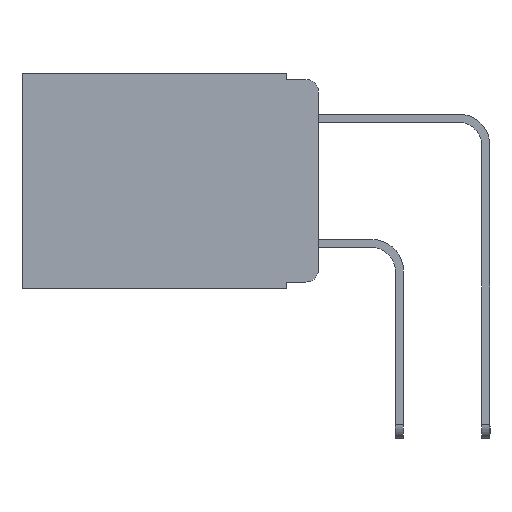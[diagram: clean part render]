
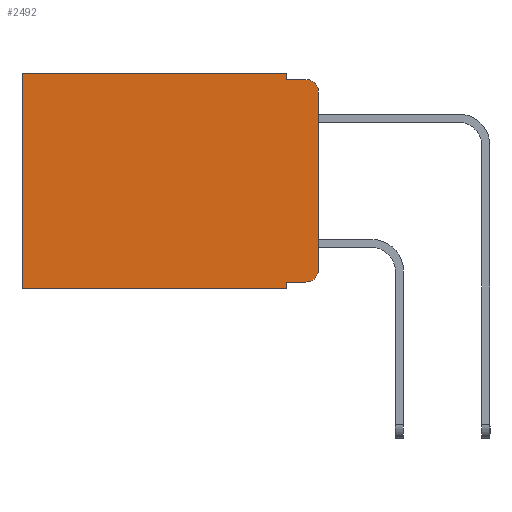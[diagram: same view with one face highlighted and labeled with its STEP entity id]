
A CAD part, left-side view. The second image highlights one B-rep face of the part: STEP entity #2492.
In plain terms, the highlighted planar face has unit normal (-1, 0, 0).
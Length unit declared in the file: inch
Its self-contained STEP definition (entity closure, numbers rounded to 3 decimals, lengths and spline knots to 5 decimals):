
#73 = ORIENTED_EDGE ( 'NONE', *, *, #131, .T. ) ;
#131 = EDGE_CURVE ( 'NONE', #2757, #17905, #5241, .T. ) ;
#643 = ORIENTED_EDGE ( 'NONE', *, *, #13208, .F. ) ;
#652 = CIRCLE ( 'NONE', #2332, 0.02 ) ;
#674 = VECTOR ( 'NONE', #5811, 39.37008 ) ;
#1659 = DIRECTION ( 'NONE',  ( 0., 0., -1. ) ) ;
#1940 = CARTESIAN_POINT ( 'NONE',  ( 0.298, 0.473, -0.343 ) ) ;
#2267 = ORIENTED_EDGE ( 'NONE', *, *, #25690, .F. ) ;
#2271 = ORIENTED_EDGE ( 'NONE', *, *, #12201, .T. ) ;
#2332 = AXIS2_PLACEMENT_3D ( 'NONE', #17751, #13495, #1659 ) ;
#2370 = ORIENTED_EDGE ( 'NONE', *, *, #26074, .T. ) ;
#2492 = ADVANCED_FACE ( 'NONE', ( #12790 ), #24912, .F. ) ;
#2679 = VERTEX_POINT ( 'NONE', #11055 ) ;
#2757 = VERTEX_POINT ( 'NONE', #25828 ) ;
#3081 = LINE ( 'NONE', #25718, #4951 ) ;
#3524 = VERTEX_POINT ( 'NONE', #13627 ) ;
#3707 = LINE ( 'NONE', #10097, #674 ) ;
#3813 = VECTOR ( 'NONE', #19562, 39.37008 ) ;
#3840 = CARTESIAN_POINT ( 'NONE',  ( 0.298, 0.051, -0.333 ) ) ;
#4006 = VECTOR ( 'NONE', #13855, 39.37008 ) ;
#4181 = CARTESIAN_POINT ( 'NONE',  ( 0.298, 0.051, -0.01 ) ) ;
#4200 = DIRECTION ( 'NONE',  ( 0., 0., -1. ) ) ;
#4491 = CARTESIAN_POINT ( 'NONE',  ( 0.298, 0.473, 0. ) ) ;
#4763 = ORIENTED_EDGE ( 'NONE', *, *, #23889, .T. ) ;
#4906 = VERTEX_POINT ( 'NONE', #18276 ) ;
#4951 = VECTOR ( 'NONE', #15460, 39.37008 ) ;
#5241 = CIRCLE ( 'NONE', #12048, 0.02 ) ;
#5261 = VERTEX_POINT ( 'NONE', #17193 ) ;
#5307 = DIRECTION ( 'NONE',  ( 0., -1., 0. ) ) ;
#5318 = CARTESIAN_POINT ( 'NONE',  ( 0.298, 0., 0. ) ) ;
#5376 = VECTOR ( 'NONE', #26197, 39.37008 ) ;
#5811 = DIRECTION ( 'NONE',  ( 0., 0., -1. ) ) ;
#6553 = DIRECTION ( 'NONE',  ( 0., 0., -1. ) ) ;
#6573 = VECTOR ( 'NONE', #4200, 39.37008 ) ;
#6792 = DIRECTION ( 'NONE',  ( 0., 0., -1. ) ) ;
#8176 = ORIENTED_EDGE ( 'NONE', *, *, #17721, .F. ) ;
#9844 = LINE ( 'NONE', #11835, #5376 ) ;
#10097 = CARTESIAN_POINT ( 'NONE',  ( 0.298, 0.473, 0. ) ) ;
#10680 = EDGE_CURVE ( 'NONE', #5261, #25159, #17855, .T. ) ;
#10824 = CARTESIAN_POINT ( 'NONE',  ( 0.298, 0.02, -0.03 ) ) ;
#10965 = VERTEX_POINT ( 'NONE', #3840 ) ;
#11055 = CARTESIAN_POINT ( 'NONE',  ( 0.298, 0.051, -0.343 ) ) ;
#11557 = ORIENTED_EDGE ( 'NONE', *, *, #10680, .T. ) ;
#11835 = CARTESIAN_POINT ( 'NONE',  ( 0.298, 0.051, 0. ) ) ;
#12042 = LINE ( 'NONE', #22428, #6573 ) ;
#12048 = AXIS2_PLACEMENT_3D ( 'NONE', #10824, #18671, #6553 ) ;
#12201 = EDGE_CURVE ( 'NONE', #25159, #25453, #3707, .T. ) ;
#12294 = DIRECTION ( 'NONE',  ( 0., -1., 0. ) ) ;
#12790 = FACE_OUTER_BOUND ( 'NONE', #15069, .T. ) ;
#13208 = EDGE_CURVE ( 'NONE', #19715, #17905, #16166, .T. ) ;
#13495 = DIRECTION ( 'NONE',  ( -1., 0., 0. ) ) ;
#13515 = EDGE_CURVE ( 'NONE', #5261, #19715, #9844, .T. ) ;
#13563 = ORIENTED_EDGE ( 'NONE', *, *, #23654, .F. ) ;
#13627 = CARTESIAN_POINT ( 'NONE',  ( 0.298, 0.02, -0.333 ) ) ;
#13760 = AXIS2_PLACEMENT_3D ( 'NONE', #14506, #22516, #6792 ) ;
#13855 = DIRECTION ( 'NONE',  ( 0., 1., 0. ) ) ;
#14506 = CARTESIAN_POINT ( 'NONE',  ( 0.298, 0., 0. ) ) ;
#15069 = EDGE_LOOP ( 'NONE', ( #8176, #73, #643, #17432, #11557, #2271, #2267, #13563, #2370, #4763 ) ) ;
#15460 = DIRECTION ( 'NONE',  ( 0., 1., 0. ) ) ;
#16166 = LINE ( 'NONE', #4181, #18551 ) ;
#17193 = CARTESIAN_POINT ( 'NONE',  ( 0.298, 0.051, 0. ) ) ;
#17432 = ORIENTED_EDGE ( 'NONE', *, *, #13515, .F. ) ;
#17560 = CARTESIAN_POINT ( 'NONE',  ( 0.298, 0.051, -0.333 ) ) ;
#17721 = EDGE_CURVE ( 'NONE', #2757, #4906, #19683, .T. ) ;
#17751 = CARTESIAN_POINT ( 'NONE',  ( 0.298, 0.02, -0.313 ) ) ;
#17855 = LINE ( 'NONE', #23987, #4006 ) ;
#17905 = VERTEX_POINT ( 'NONE', #22087 ) ;
#18276 = CARTESIAN_POINT ( 'NONE',  ( 0.298, 0., -0.313 ) ) ;
#18551 = VECTOR ( 'NONE', #12294, 39.37008 ) ;
#18671 = DIRECTION ( 'NONE',  ( -1., 0., 0. ) ) ;
#19562 = DIRECTION ( 'NONE',  ( 0., 0., -1. ) ) ;
#19683 = LINE ( 'NONE', #5318, #3813 ) ;
#19715 = VERTEX_POINT ( 'NONE', #21722 ) ;
#21549 = LINE ( 'NONE', #17560, #25815 ) ;
#21722 = CARTESIAN_POINT ( 'NONE',  ( 0.298, 0.051, -0.01 ) ) ;
#22087 = CARTESIAN_POINT ( 'NONE',  ( 0.298, 0.02, -0.01 ) ) ;
#22428 = CARTESIAN_POINT ( 'NONE',  ( 0.298, 0.051, 0. ) ) ;
#22516 = DIRECTION ( 'NONE',  ( 1., 0., 0. ) ) ;
#23654 = EDGE_CURVE ( 'NONE', #10965, #2679, #12042, .T. ) ;
#23889 = EDGE_CURVE ( 'NONE', #3524, #4906, #652, .T. ) ;
#23987 = CARTESIAN_POINT ( 'NONE',  ( 0.298, 0., 0. ) ) ;
#24912 = PLANE ( 'NONE',  #13760 ) ;
#25159 = VERTEX_POINT ( 'NONE', #4491 ) ;
#25453 = VERTEX_POINT ( 'NONE', #1940 ) ;
#25690 = EDGE_CURVE ( 'NONE', #2679, #25453, #3081, .T. ) ;
#25718 = CARTESIAN_POINT ( 'NONE',  ( 0.298, 0., -0.343 ) ) ;
#25815 = VECTOR ( 'NONE', #5307, 39.37008 ) ;
#25828 = CARTESIAN_POINT ( 'NONE',  ( 0.298, 0., -0.03 ) ) ;
#26074 = EDGE_CURVE ( 'NONE', #10965, #3524, #21549, .T. ) ;
#26197 = DIRECTION ( 'NONE',  ( 0., 0., -1. ) ) ;
